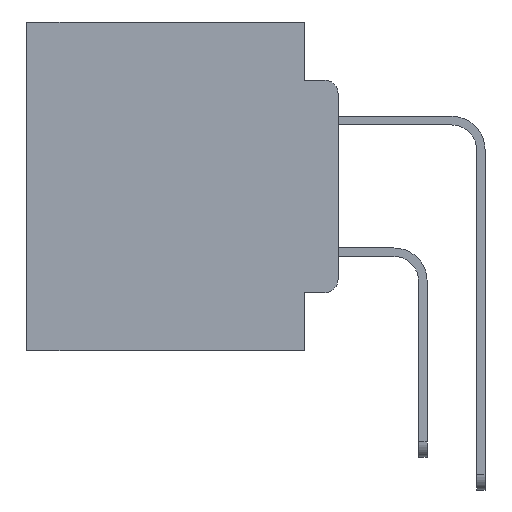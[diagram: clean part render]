
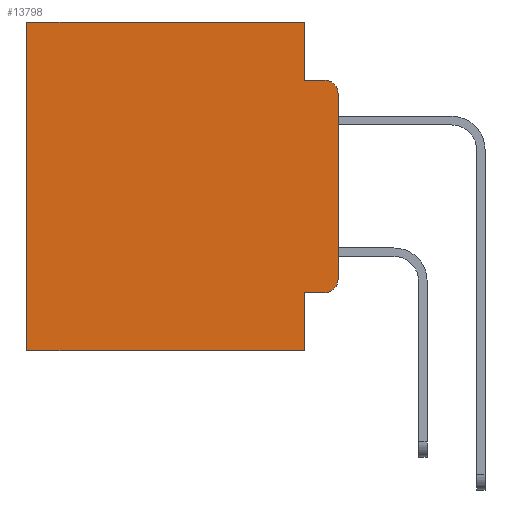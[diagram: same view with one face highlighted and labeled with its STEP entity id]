
A CAD part, left-side view. The second image highlights one B-rep face of the part: STEP entity #13798.
In plain terms, the highlighted planar face has unit normal (-1, 0, 0).
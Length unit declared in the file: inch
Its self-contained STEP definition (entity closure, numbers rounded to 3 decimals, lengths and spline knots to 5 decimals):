
#1060 = CARTESIAN_POINT ( 'NONE',  ( 0.298, 0., 0. ) ) ;
#1574 = VERTEX_POINT ( 'NONE', #24453 ) ;
#1852 = DIRECTION ( 'NONE',  ( 0., 1., 0. ) ) ;
#1891 = AXIS2_PLACEMENT_3D ( 'NONE', #1060, #23445, #10284 ) ;
#1904 = ORIENTED_EDGE ( 'NONE', *, *, #5921, .T. ) ;
#2646 = EDGE_CURVE ( 'NONE', #3931, #18808, #5007, .T. ) ;
#2699 = LINE ( 'NONE', #6469, #8759 ) ;
#2819 = EDGE_CURVE ( 'NONE', #24286, #18808, #23747, .T. ) ;
#3282 = ORIENTED_EDGE ( 'NONE', *, *, #8925, .T. ) ;
#3402 = PLANE ( 'NONE',  #1891 ) ;
#3414 = VERTEX_POINT ( 'NONE', #24287 ) ;
#3594 = DIRECTION ( 'NONE',  ( 0., -1., 0. ) ) ;
#3931 = VERTEX_POINT ( 'NONE', #12873 ) ;
#5007 = LINE ( 'NONE', #22512, #22732 ) ;
#5865 = LINE ( 'NONE', #25739, #11196 ) ;
#5866 = EDGE_CURVE ( 'NONE', #17727, #19153, #16098, .T. ) ;
#5921 = EDGE_CURVE ( 'NONE', #17727, #24286, #2699, .T. ) ;
#6469 = CARTESIAN_POINT ( 'NONE',  ( 0.298, 0., 0. ) ) ;
#6509 = ORIENTED_EDGE ( 'NONE', *, *, #2819, .T. ) ;
#6522 = DIRECTION ( 'NONE',  ( 0., 0., -1. ) ) ;
#6775 = DIRECTION ( 'NONE',  ( -1., 0., 0. ) ) ;
#7193 = ORIENTED_EDGE ( 'NONE', *, *, #25707, .F. ) ;
#7395 = EDGE_CURVE ( 'NONE', #19153, #11375, #18777, .T. ) ;
#8759 = VECTOR ( 'NONE', #1852, 39.37008 ) ;
#8925 = EDGE_CURVE ( 'NONE', #1574, #11375, #20195, .T. ) ;
#9317 = CARTESIAN_POINT ( 'NONE',  ( 0.298, 0., 0. ) ) ;
#9406 = CARTESIAN_POINT ( 'NONE',  ( 0.298, 0.051, -0.4115 ) ) ;
#9902 = FACE_OUTER_BOUND ( 'NONE', #16881, .T. ) ;
#10284 = DIRECTION ( 'NONE',  ( 0., 0., -1. ) ) ;
#10846 = CARTESIAN_POINT ( 'NONE',  ( 0.298, 0.051, 0. ) ) ;
#11196 = VECTOR ( 'NONE', #14875, 39.37008 ) ;
#11375 = VERTEX_POINT ( 'NONE', #17077 ) ;
#12873 = CARTESIAN_POINT ( 'NONE',  ( 0.298, 0.051, -0.5 ) ) ;
#13235 = DIRECTION ( 'NONE',  ( -1., 0., 0. ) ) ;
#13798 = ADVANCED_FACE ( 'NONE', ( #9902 ), #3402, .F. ) ;
#13926 = LINE ( 'NONE', #19856, #25564 ) ;
#14875 = DIRECTION ( 'NONE',  ( 0., -1., 0. ) ) ;
#14944 = EDGE_CURVE ( 'NONE', #1574, #16090, #26278, .T. ) ;
#15419 = VECTOR ( 'NONE', #28385, 39.37008 ) ;
#15472 = CIRCLE ( 'NONE', #18508, 0.02 ) ;
#16089 = CARTESIAN_POINT ( 'NONE',  ( 0.298, 0., -0.3915 ) ) ;
#16090 = VERTEX_POINT ( 'NONE', #16089 ) ;
#16098 = LINE ( 'NONE', #10846, #15419 ) ;
#16881 = EDGE_LOOP ( 'NONE', ( #28590, #3282, #22445, #22819, #1904, #6509, #19031, #7193, #25535, #19417 ) ) ;
#17077 = CARTESIAN_POINT ( 'NONE',  ( 0.298, 0.02, -0.0885 ) ) ;
#17095 = CARTESIAN_POINT ( 'NONE',  ( 0.298, 0.051, -0.0885 ) ) ;
#17120 = CARTESIAN_POINT ( 'NONE',  ( 0.298, 0.473, 0. ) ) ;
#17272 = CARTESIAN_POINT ( 'NONE',  ( 0.298, 0.473, 0. ) ) ;
#17311 = VECTOR ( 'NONE', #17642, 39.37008 ) ;
#17642 = DIRECTION ( 'NONE',  ( 0., 0., -1. ) ) ;
#17661 = CARTESIAN_POINT ( 'NONE',  ( 0.298, 0.473, -0.5 ) ) ;
#17727 = VERTEX_POINT ( 'NONE', #20384 ) ;
#18508 = AXIS2_PLACEMENT_3D ( 'NONE', #20093, #6775, #22254 ) ;
#18777 = LINE ( 'NONE', #17095, #25242 ) ;
#18808 = VERTEX_POINT ( 'NONE', #17661 ) ;
#18922 = AXIS2_PLACEMENT_3D ( 'NONE', #26341, #13235, #28531 ) ;
#19031 = ORIENTED_EDGE ( 'NONE', *, *, #2646, .F. ) ;
#19153 = VERTEX_POINT ( 'NONE', #19349 ) ;
#19349 = CARTESIAN_POINT ( 'NONE',  ( 0.298, 0.051, -0.0885 ) ) ;
#19417 = ORIENTED_EDGE ( 'NONE', *, *, #22755, .T. ) ;
#19856 = CARTESIAN_POINT ( 'NONE',  ( 0.298, 0.051, 0. ) ) ;
#20093 = CARTESIAN_POINT ( 'NONE',  ( 0.298, 0.02, -0.3915 ) ) ;
#20195 = CIRCLE ( 'NONE', #18922, 0.02 ) ;
#20384 = CARTESIAN_POINT ( 'NONE',  ( 0.298, 0.051, 0. ) ) ;
#20489 = VECTOR ( 'NONE', #26916, 39.37008 ) ;
#21678 = VERTEX_POINT ( 'NONE', #9406 ) ;
#22254 = DIRECTION ( 'NONE',  ( 0., 0., -1. ) ) ;
#22445 = ORIENTED_EDGE ( 'NONE', *, *, #7395, .F. ) ;
#22512 = CARTESIAN_POINT ( 'NONE',  ( 0.298, 0., -0.5 ) ) ;
#22732 = VECTOR ( 'NONE', #23162, 39.37008 ) ;
#22755 = EDGE_CURVE ( 'NONE', #3414, #16090, #15472, .T. ) ;
#22819 = ORIENTED_EDGE ( 'NONE', *, *, #5866, .F. ) ;
#23162 = DIRECTION ( 'NONE',  ( 0., 1., 0. ) ) ;
#23445 = DIRECTION ( 'NONE',  ( 1., 0., 0. ) ) ;
#23747 = LINE ( 'NONE', #17120, #17311 ) ;
#24232 = EDGE_CURVE ( 'NONE', #21678, #3414, #5865, .T. ) ;
#24286 = VERTEX_POINT ( 'NONE', #17272 ) ;
#24287 = CARTESIAN_POINT ( 'NONE',  ( 0.298, 0.02, -0.4115 ) ) ;
#24453 = CARTESIAN_POINT ( 'NONE',  ( 0.298, 0., -0.1085 ) ) ;
#25242 = VECTOR ( 'NONE', #3594, 39.37008 ) ;
#25535 = ORIENTED_EDGE ( 'NONE', *, *, #24232, .T. ) ;
#25564 = VECTOR ( 'NONE', #6522, 39.37008 ) ;
#25707 = EDGE_CURVE ( 'NONE', #21678, #3931, #13926, .T. ) ;
#25739 = CARTESIAN_POINT ( 'NONE',  ( 0.298, 0.051, -0.4115 ) ) ;
#26278 = LINE ( 'NONE', #9317, #20489 ) ;
#26341 = CARTESIAN_POINT ( 'NONE',  ( 0.298, 0.02, -0.1085 ) ) ;
#26916 = DIRECTION ( 'NONE',  ( 0., 0., -1. ) ) ;
#28385 = DIRECTION ( 'NONE',  ( 0., 0., -1. ) ) ;
#28531 = DIRECTION ( 'NONE',  ( 0., 0., -1. ) ) ;
#28590 = ORIENTED_EDGE ( 'NONE', *, *, #14944, .F. ) ;
